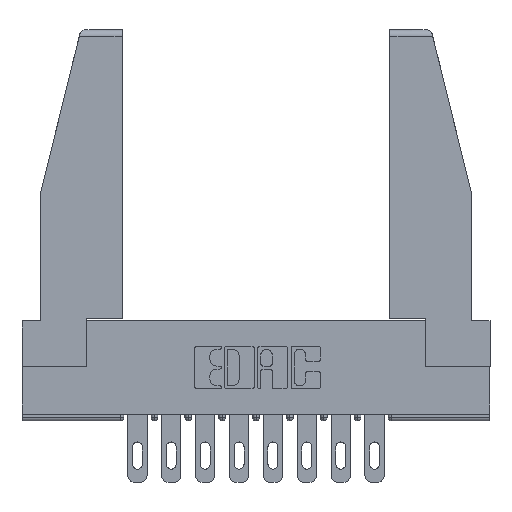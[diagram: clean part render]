
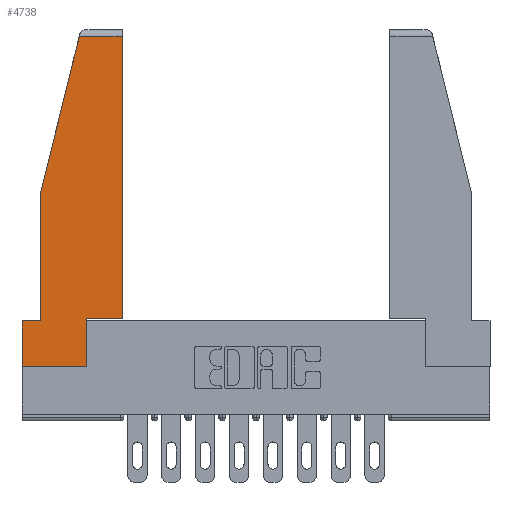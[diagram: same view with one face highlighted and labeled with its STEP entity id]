
A CAD part, top view. The second image highlights one B-rep face of the part: STEP entity #4738.
In plain terms, the highlighted planar face has unit normal (0, 0, 1).
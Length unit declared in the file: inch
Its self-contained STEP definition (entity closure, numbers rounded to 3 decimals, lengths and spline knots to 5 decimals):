
#105 = EDGE_CURVE ( 'NONE', #9670, #15243, #12337, .T. ) ;
#158 = EDGE_LOOP ( 'NONE', ( #1858, #12145, #4419, #7950, #8583, #2527, #8142, #14294, #6470 ) ) ;
#468 = EDGE_CURVE ( 'NONE', #2286, #14229, #6557, .T. ) ;
#522 = EDGE_CURVE ( 'NONE', #10045, #6745, #4351, .T. ) ;
#774 = CARTESIAN_POINT ( 'NONE',  ( 0.086, 0.8, 0. ) ) ;
#831 = DIRECTION ( 'NONE',  ( -1., 0., 0. ) ) ;
#912 = CARTESIAN_POINT ( 'NONE',  ( 0.461, 0.223, 0. ) ) ;
#1805 = LINE ( 'NONE', #13751, #13970 ) ;
#1858 = ORIENTED_EDGE ( 'NONE', *, *, #522, .T. ) ;
#2085 = VECTOR ( 'NONE', #831, 39.37008 ) ;
#2286 = VERTEX_POINT ( 'NONE', #4143 ) ;
#2527 = ORIENTED_EDGE ( 'NONE', *, *, #9683, .T. ) ;
#2687 = EDGE_CURVE ( 'NONE', #4033, #14408, #14256, .T. ) ;
#2910 = EDGE_CURVE ( 'NONE', #6745, #2286, #6479, .T. ) ;
#3081 = PLANE ( 'NONE',  #6260 ) ;
#3968 = EDGE_CURVE ( 'NONE', #14408, #11125, #13487, .T. ) ;
#4033 = VERTEX_POINT ( 'NONE', #9144 ) ;
#4143 = CARTESIAN_POINT ( 'NONE',  ( 0.2636, 1.52, 0. ) ) ;
#4252 = CARTESIAN_POINT ( 'NONE',  ( 0., 0., 0. ) ) ;
#4351 = LINE ( 'NONE', #13038, #9165 ) ;
#4368 = VECTOR ( 'NONE', #6242, 39.37008 ) ;
#4419 = ORIENTED_EDGE ( 'NONE', *, *, #468, .T. ) ;
#4454 = CARTESIAN_POINT ( 'NONE',  ( 0.297, 0., 0. ) ) ;
#4682 = FACE_OUTER_BOUND ( 'NONE', #158, .T. ) ;
#4738 = ADVANCED_FACE ( 'NONE', ( #4682 ), #3081, .T. ) ;
#5814 = EDGE_CURVE ( 'NONE', #11125, #10045, #14993, .T. ) ;
#6242 = DIRECTION ( 'NONE',  ( -1., 0., 0. ) ) ;
#6260 = AXIS2_PLACEMENT_3D ( 'NONE', #4252, #13604, #13652 ) ;
#6470 = ORIENTED_EDGE ( 'NONE', *, *, #5814, .T. ) ;
#6479 = LINE ( 'NONE', #8014, #2085 ) ;
#6557 = LINE ( 'NONE', #10764, #10649 ) ;
#6709 = CARTESIAN_POINT ( 'NONE',  ( 0.086, 0.21, 0. ) ) ;
#6740 = DIRECTION ( 'NONE',  ( 0., 1., 0. ) ) ;
#6745 = VERTEX_POINT ( 'NONE', #11232 ) ;
#7076 = CARTESIAN_POINT ( 'NONE',  ( 0.297, 0.223, 0. ) ) ;
#7162 = CARTESIAN_POINT ( 'NONE',  ( 0.086, 0.8, 0. ) ) ;
#7196 = VECTOR ( 'NONE', #6740, 39.37008 ) ;
#7273 = CARTESIAN_POINT ( 'NONE',  ( 0., 0., 0. ) ) ;
#7950 = ORIENTED_EDGE ( 'NONE', *, *, #10987, .T. ) ;
#8014 = CARTESIAN_POINT ( 'NONE',  ( 0., 1.52, 0. ) ) ;
#8142 = ORIENTED_EDGE ( 'NONE', *, *, #2687, .T. ) ;
#8329 = DIRECTION ( 'NONE',  ( 0., 1., 0. ) ) ;
#8583 = ORIENTED_EDGE ( 'NONE', *, *, #105, .T. ) ;
#9144 = CARTESIAN_POINT ( 'NONE',  ( 0., 0., 0. ) ) ;
#9165 = VECTOR ( 'NONE', #8329, 39.37008 ) ;
#9196 = CARTESIAN_POINT ( 'NONE',  ( 0.297, 0., 0. ) ) ;
#9272 = VECTOR ( 'NONE', #11579, 39.37008 ) ;
#9670 = VERTEX_POINT ( 'NONE', #6709 ) ;
#9683 = EDGE_CURVE ( 'NONE', #15243, #4033, #1805, .T. ) ;
#10045 = VERTEX_POINT ( 'NONE', #912 ) ;
#10405 = DIRECTION ( 'NONE',  ( 0., -1., 0. ) ) ;
#10649 = VECTOR ( 'NONE', #12889, 39.37008 ) ;
#10676 = LINE ( 'NONE', #774, #13450 ) ;
#10764 = CARTESIAN_POINT ( 'NONE',  ( 0.271, 1.55, 0. ) ) ;
#10782 = CARTESIAN_POINT ( 'NONE',  ( 0., 0.21, 0. ) ) ;
#10987 = EDGE_CURVE ( 'NONE', #14229, #9670, #10676, .T. ) ;
#11125 = VERTEX_POINT ( 'NONE', #7076 ) ;
#11232 = CARTESIAN_POINT ( 'NONE',  ( 0.461, 1.52, 0. ) ) ;
#11579 = DIRECTION ( 'NONE',  ( 1., 0., 0. ) ) ;
#12145 = ORIENTED_EDGE ( 'NONE', *, *, #2910, .T. ) ;
#12337 = LINE ( 'NONE', #10782, #4368 ) ;
#12587 = VECTOR ( 'NONE', #13275, 39.37008 ) ;
#12889 = DIRECTION ( 'NONE',  ( -0.239, -0.971, 0. ) ) ;
#12969 = CARTESIAN_POINT ( 'NONE',  ( 0.297, 0.223, 0. ) ) ;
#13038 = CARTESIAN_POINT ( 'NONE',  ( 0.461, 0.223, 0. ) ) ;
#13275 = DIRECTION ( 'NONE',  ( 1., 0., 0. ) ) ;
#13404 = CARTESIAN_POINT ( 'NONE',  ( 0., 0.21, 0. ) ) ;
#13450 = VECTOR ( 'NONE', #15202, 39.37008 ) ;
#13487 = LINE ( 'NONE', #9196, #7196 ) ;
#13604 = DIRECTION ( 'NONE',  ( 0., 0., 1. ) ) ;
#13652 = DIRECTION ( 'NONE',  ( 1., 0., 0. ) ) ;
#13751 = CARTESIAN_POINT ( 'NONE',  ( 0., 0.21, 0. ) ) ;
#13970 = VECTOR ( 'NONE', #10405, 39.37008 ) ;
#14229 = VERTEX_POINT ( 'NONE', #7162 ) ;
#14256 = LINE ( 'NONE', #7273, #12587 ) ;
#14294 = ORIENTED_EDGE ( 'NONE', *, *, #3968, .T. ) ;
#14408 = VERTEX_POINT ( 'NONE', #4454 ) ;
#14993 = LINE ( 'NONE', #12969, #9272 ) ;
#15202 = DIRECTION ( 'NONE',  ( 0., -1., 0. ) ) ;
#15243 = VERTEX_POINT ( 'NONE', #13404 ) ;
